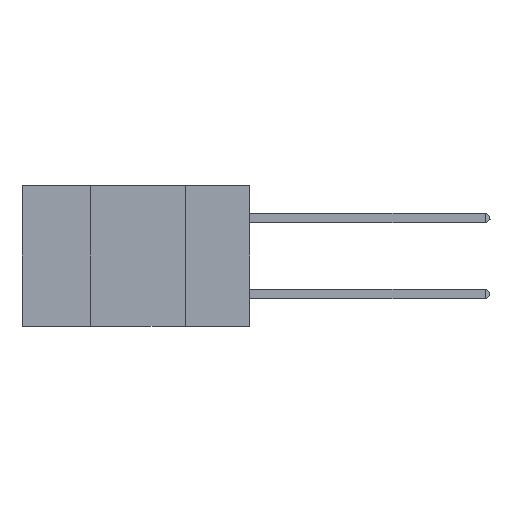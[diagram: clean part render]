
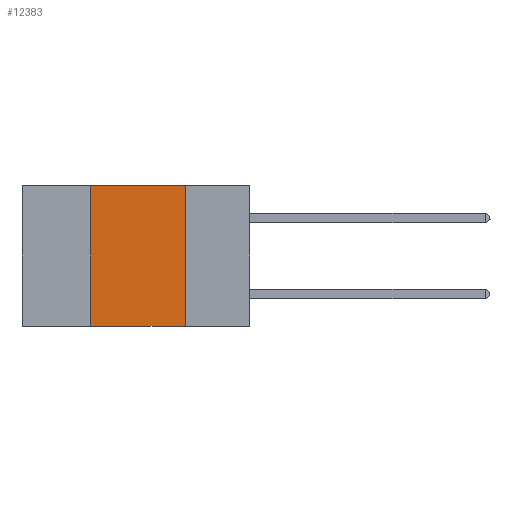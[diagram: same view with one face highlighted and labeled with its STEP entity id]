
A CAD part, left-side view. The second image highlights one B-rep face of the part: STEP entity #12383.
In plain terms, the highlighted planar face has unit normal (-1, 0, 0).
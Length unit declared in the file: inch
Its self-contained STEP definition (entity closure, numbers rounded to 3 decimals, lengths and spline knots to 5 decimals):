
#214 = DIRECTION ( 'NONE',  ( 0., -1., 0. ) ) ;
#724 = VECTOR ( 'NONE', #8394, 39.37008 ) ;
#1295 = DIRECTION ( 'NONE',  ( 0., -1., 0. ) ) ;
#1840 = ORIENTED_EDGE ( 'NONE', *, *, #13233, .T. ) ;
#2252 = CARTESIAN_POINT ( 'NONE',  ( 0., 0.6, 0. ) ) ;
#2386 = LINE ( 'NONE', #2482, #16091 ) ;
#2449 = VERTEX_POINT ( 'NONE', #7263 ) ;
#2482 = CARTESIAN_POINT ( 'NONE',  ( 0., 0.6, 0. ) ) ;
#2778 = DIRECTION ( 'NONE',  ( 0., 0., 1. ) ) ;
#4160 = VERTEX_POINT ( 'NONE', #13460 ) ;
#4174 = AXIS2_PLACEMENT_3D ( 'NONE', #2252, #13118, #14568 ) ;
#4576 = CARTESIAN_POINT ( 'NONE',  ( 0., 0.17, 0. ) ) ;
#4849 = ORIENTED_EDGE ( 'NONE', *, *, #15867, .F. ) ;
#5290 = LINE ( 'NONE', #14991, #6867 ) ;
#5737 = EDGE_LOOP ( 'NONE', ( #5869, #11174, #4849, #1840 ) ) ;
#5869 = ORIENTED_EDGE ( 'NONE', *, *, #11260, .F. ) ;
#6867 = VECTOR ( 'NONE', #2778, 39.37008 ) ;
#7263 = CARTESIAN_POINT ( 'NONE',  ( 0., 0.42, 0. ) ) ;
#7585 = PLANE ( 'NONE',  #4174 ) ;
#8192 = VERTEX_POINT ( 'NONE', #10117 ) ;
#8394 = DIRECTION ( 'NONE',  ( 0., 0., -1. ) ) ;
#8706 = CARTESIAN_POINT ( 'NONE',  ( 0., 0.17, -0.37 ) ) ;
#9026 = FACE_OUTER_BOUND ( 'NONE', #5737, .T. ) ;
#10117 = CARTESIAN_POINT ( 'NONE',  ( 0., 0.17, 0. ) ) ;
#11174 = ORIENTED_EDGE ( 'NONE', *, *, #13435, .F. ) ;
#11201 = LINE ( 'NONE', #16750, #17553 ) ;
#11260 = EDGE_CURVE ( 'NONE', #8192, #15029, #16861, .T. ) ;
#12383 = ADVANCED_FACE ( 'NONE', ( #9026 ), #7585, .F. ) ;
#13118 = DIRECTION ( 'NONE',  ( 1., 0., 0. ) ) ;
#13233 = EDGE_CURVE ( 'NONE', #4160, #15029, #11201, .T. ) ;
#13435 = EDGE_CURVE ( 'NONE', #2449, #8192, #2386, .T. ) ;
#13460 = CARTESIAN_POINT ( 'NONE',  ( 0., 0.42, -0.37 ) ) ;
#14568 = DIRECTION ( 'NONE',  ( 0., 0., -1. ) ) ;
#14991 = CARTESIAN_POINT ( 'NONE',  ( 0., 0.42, 0. ) ) ;
#15029 = VERTEX_POINT ( 'NONE', #8706 ) ;
#15867 = EDGE_CURVE ( 'NONE', #4160, #2449, #5290, .T. ) ;
#16091 = VECTOR ( 'NONE', #1295, 39.37008 ) ;
#16750 = CARTESIAN_POINT ( 'NONE',  ( 0., 0.6, -0.37 ) ) ;
#16861 = LINE ( 'NONE', #4576, #724 ) ;
#17553 = VECTOR ( 'NONE', #214, 39.37008 ) ;
